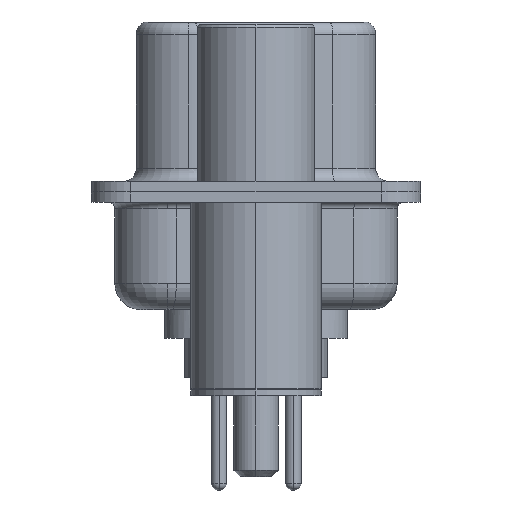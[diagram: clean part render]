
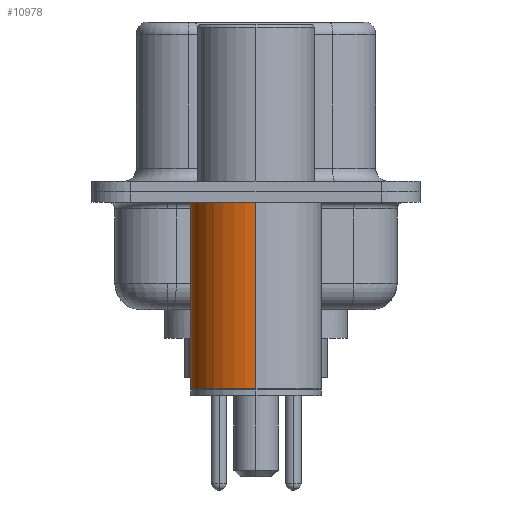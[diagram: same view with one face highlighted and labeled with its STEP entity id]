
A CAD part, left-side view. The second image highlights one B-rep face of the part: STEP entity #10978.
In plain terms, the highlighted cylindrical face has radius 2.5 mm (diameter 5 mm), a partial arc.
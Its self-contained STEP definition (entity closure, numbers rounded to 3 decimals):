
#635 = EDGE_LOOP ( 'NONE', ( #6937, #12218, #13108, #14647 ) ) ;
#984 = CARTESIAN_POINT ( 'NONE',  ( -2.5, 0., -0.4 ) ) ;
#1092 = EDGE_CURVE ( 'NONE', #3666, #12681, #16533, .T. ) ;
#2261 = EDGE_CURVE ( 'NONE', #23208, #10955, #20824, .T. ) ;
#3319 = DIRECTION ( 'NONE',  ( 0., 0., 1. ) ) ;
#3666 = VERTEX_POINT ( 'NONE', #13049 ) ;
#4586 = CARTESIAN_POINT ( 'NONE',  ( -2.5, 0., 0.581 ) ) ;
#4674 = DIRECTION ( 'NONE',  ( 1., 0., 0. ) ) ;
#4829 = CARTESIAN_POINT ( 'NONE',  ( 0., 0., 0.581 ) ) ;
#5513 = CARTESIAN_POINT ( 'NONE',  ( 0., 0., -7.525 ) ) ;
#5569 = LINE ( 'NONE', #9244, #19948 ) ;
#6487 = DIRECTION ( 'NONE',  ( 0., 0., 1. ) ) ;
#6740 = DIRECTION ( 'NONE',  ( 1., 0., 0. ) ) ;
#6937 = ORIENTED_EDGE ( 'NONE', *, *, #1092, .T. ) ;
#9180 = AXIS2_PLACEMENT_3D ( 'NONE', #4829, #14225, #6740 ) ;
#9244 = CARTESIAN_POINT ( 'NONE',  ( 2.5, 0., 0.581 ) ) ;
#9594 = FACE_OUTER_BOUND ( 'NONE', #635, .T. ) ;
#10955 = VERTEX_POINT ( 'NONE', #984 ) ;
#10978 = ADVANCED_FACE ( 'NONE', ( #9594 ), #13980, .T. ) ;
#12218 = ORIENTED_EDGE ( 'NONE', *, *, #14234, .T. ) ;
#12681 = VERTEX_POINT ( 'NONE', #23897 ) ;
#13049 = CARTESIAN_POINT ( 'NONE',  ( 2.5, 0., -7.525 ) ) ;
#13108 = ORIENTED_EDGE ( 'NONE', *, *, #2261, .F. ) ;
#13313 = VECTOR ( 'NONE', #6487, 1000. ) ;
#13980 = CYLINDRICAL_SURFACE ( 'NONE', #9180, 2.5 ) ;
#14225 = DIRECTION ( 'NONE',  ( 0., 0., 1. ) ) ;
#14234 = EDGE_CURVE ( 'NONE', #12681, #10955, #18281, .T. ) ;
#14647 = ORIENTED_EDGE ( 'NONE', *, *, #15995, .F. ) ;
#15995 = EDGE_CURVE ( 'NONE', #3666, #23208, #5569, .T. ) ;
#16533 = CIRCLE ( 'NONE', #20800, 2.5 ) ;
#18281 = LINE ( 'NONE', #4586, #13313 ) ;
#18982 = AXIS2_PLACEMENT_3D ( 'NONE', #24028, #3319, #22528 ) ;
#19926 = CARTESIAN_POINT ( 'NONE',  ( 2.5, 0., -0.4 ) ) ;
#19948 = VECTOR ( 'NONE', #20401, 1000. ) ;
#20401 = DIRECTION ( 'NONE',  ( 0., 0., 1. ) ) ;
#20495 = DIRECTION ( 'NONE',  ( 0., 0., 1. ) ) ;
#20800 = AXIS2_PLACEMENT_3D ( 'NONE', #5513, #20495, #4674 ) ;
#20824 = CIRCLE ( 'NONE', #18982, 2.5 ) ;
#22528 = DIRECTION ( 'NONE',  ( 1., 0., 0. ) ) ;
#23208 = VERTEX_POINT ( 'NONE', #19926 ) ;
#23897 = CARTESIAN_POINT ( 'NONE',  ( -2.5, 0., -7.525 ) ) ;
#24028 = CARTESIAN_POINT ( 'NONE',  ( 0., 0., -0.4 ) ) ;
